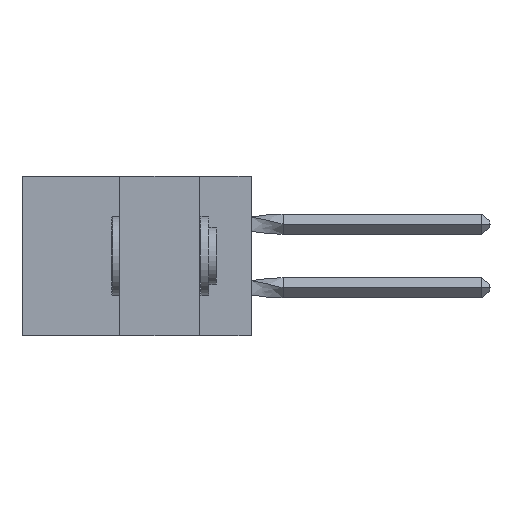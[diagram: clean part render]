
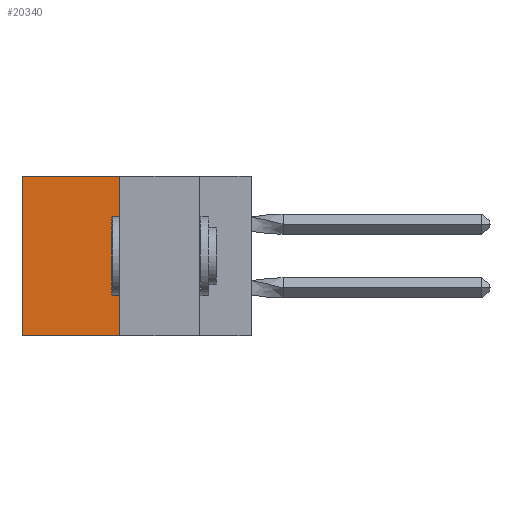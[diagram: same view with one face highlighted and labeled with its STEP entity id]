
A CAD part, left-side view. The second image highlights one B-rep face of the part: STEP entity #20340.
In plain terms, the highlighted planar face has unit normal (-1, 0, 0).
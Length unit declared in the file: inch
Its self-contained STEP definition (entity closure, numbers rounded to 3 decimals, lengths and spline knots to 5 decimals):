
#72 = CARTESIAN_POINT ( 'NONE',  ( 0.305, 0.72, -0.5 ) ) ;
#748 = ORIENTED_EDGE ( 'NONE', *, *, #9958, .T. ) ;
#2188 = ORIENTED_EDGE ( 'NONE', *, *, #25052, .T. ) ;
#4117 = CARTESIAN_POINT ( 'NONE',  ( 0.305, 0.413, 0. ) ) ;
#4361 = EDGE_CURVE ( 'NONE', #20723, #15363, #29427, .T. ) ;
#6310 = VECTOR ( 'NONE', #11230, 39.37008 ) ;
#7392 = DIRECTION ( 'NONE',  ( 1., 0., 0. ) ) ;
#7530 = CARTESIAN_POINT ( 'NONE',  ( 0.305, 0.413, -0.5 ) ) ;
#8046 = FACE_OUTER_BOUND ( 'NONE', #16745, .T. ) ;
#8836 = AXIS2_PLACEMENT_3D ( 'NONE', #19022, #7392, #12339 ) ;
#9040 = CARTESIAN_POINT ( 'NONE',  ( 0.305, 0.72, -0.5 ) ) ;
#9958 = EDGE_CURVE ( 'NONE', #20723, #18497, #26839, .T. ) ;
#11200 = DIRECTION ( 'NONE',  ( 0., 1., 0. ) ) ;
#11230 = DIRECTION ( 'NONE',  ( 0., 0., -1. ) ) ;
#12339 = DIRECTION ( 'NONE',  ( 0., 0., -1. ) ) ;
#12472 = LINE ( 'NONE', #9040, #6310 ) ;
#13110 = VECTOR ( 'NONE', #26372, 39.37008 ) ;
#13321 = ORIENTED_EDGE ( 'NONE', *, *, #4361, .F. ) ;
#14466 = PLANE ( 'NONE',  #8836 ) ;
#15363 = VERTEX_POINT ( 'NONE', #15995 ) ;
#15660 = DIRECTION ( 'NONE',  ( 0., 1., 0. ) ) ;
#15995 = CARTESIAN_POINT ( 'NONE',  ( 0.305, 0.413, -0.5 ) ) ;
#16745 = EDGE_LOOP ( 'NONE', ( #2188, #22707, #13321, #748 ) ) ;
#17602 = VECTOR ( 'NONE', #15660, 39.37008 ) ;
#18497 = VERTEX_POINT ( 'NONE', #20751 ) ;
#19022 = CARTESIAN_POINT ( 'NONE',  ( 0.305, 0.413, -0.5 ) ) ;
#20340 = ADVANCED_FACE ( 'NONE', ( #8046 ), #14466, .F. ) ;
#20723 = VERTEX_POINT ( 'NONE', #21112 ) ;
#20751 = CARTESIAN_POINT ( 'NONE',  ( 0.305, 0.72, 0. ) ) ;
#21035 = VECTOR ( 'NONE', #11200, 39.37008 ) ;
#21112 = CARTESIAN_POINT ( 'NONE',  ( 0.305, 0.413, 0. ) ) ;
#21266 = LINE ( 'NONE', #27210, #17602 ) ;
#22707 = ORIENTED_EDGE ( 'NONE', *, *, #28474, .F. ) ;
#24116 = VERTEX_POINT ( 'NONE', #72 ) ;
#25052 = EDGE_CURVE ( 'NONE', #18497, #24116, #12472, .T. ) ;
#26372 = DIRECTION ( 'NONE',  ( 0., 0., -1. ) ) ;
#26839 = LINE ( 'NONE', #4117, #21035 ) ;
#27210 = CARTESIAN_POINT ( 'NONE',  ( 0.305, 0.413, -0.5 ) ) ;
#28474 = EDGE_CURVE ( 'NONE', #15363, #24116, #21266, .T. ) ;
#29427 = LINE ( 'NONE', #7530, #13110 ) ;
